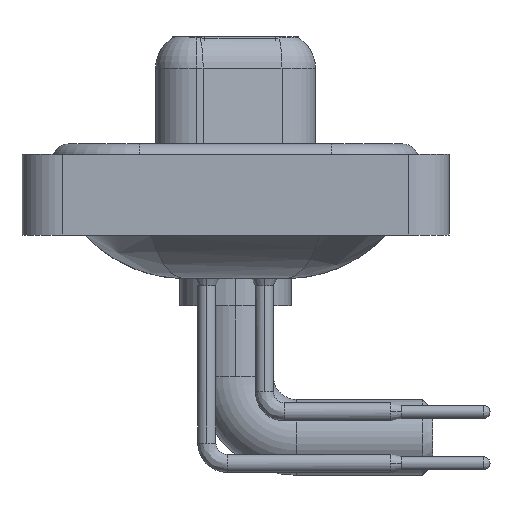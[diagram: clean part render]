
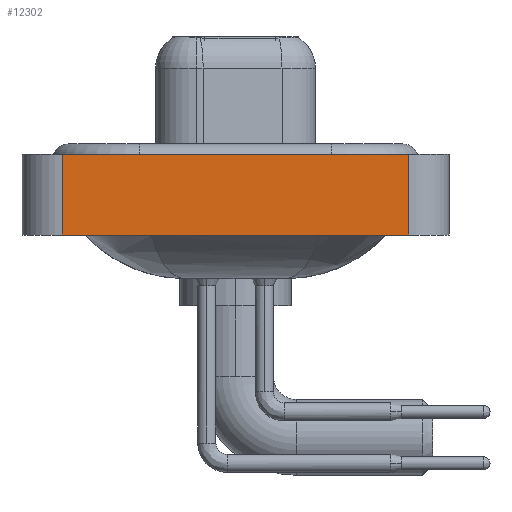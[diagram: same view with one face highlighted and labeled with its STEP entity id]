
A CAD part, left-side view. The second image highlights one B-rep face of the part: STEP entity #12302.
In plain terms, the highlighted planar face has unit normal (-1, 0, 0).
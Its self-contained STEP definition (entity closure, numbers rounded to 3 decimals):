
#582 = CARTESIAN_POINT ( 'NONE',  ( -7.3, 8.55, 0.4 ) ) ;
#676 = DIRECTION ( 'NONE',  ( -1., 0., 0. ) ) ;
#2109 = VERTEX_POINT ( 'NONE', #6338 ) ;
#2579 = LINE ( 'NONE', #5613, #11020 ) ;
#2845 = CARTESIAN_POINT ( 'NONE',  ( -7.3, 8.55, -3.6 ) ) ;
#2897 = CARTESIAN_POINT ( 'NONE',  ( -7.3, 8.55, -3.6 ) ) ;
#2934 = EDGE_CURVE ( 'NONE', #4146, #2109, #2579, .T. ) ;
#4146 = VERTEX_POINT ( 'NONE', #8092 ) ;
#4846 = EDGE_LOOP ( 'NONE', ( #12628, #10333, #7640, #14711 ) ) ;
#5613 = CARTESIAN_POINT ( 'NONE',  ( -7.3, -8.55, -3.6 ) ) ;
#5783 = VERTEX_POINT ( 'NONE', #582 ) ;
#6338 = CARTESIAN_POINT ( 'NONE',  ( -7.3, -8.55, 0.4 ) ) ;
#6369 = VECTOR ( 'NONE', #18248, 1000. ) ;
#7221 = DIRECTION ( 'NONE',  ( 0., -1., 0. ) ) ;
#7640 = ORIENTED_EDGE ( 'NONE', *, *, #9861, .F. ) ;
#8092 = CARTESIAN_POINT ( 'NONE',  ( -7.3, -8.55, -3.6 ) ) ;
#9240 = PLANE ( 'NONE',  #22042 ) ;
#9298 = LINE ( 'NONE', #19200, #12912 ) ;
#9682 = VECTOR ( 'NONE', #7221, 1000. ) ;
#9861 = EDGE_CURVE ( 'NONE', #12915, #5783, #14653, .T. ) ;
#10333 = ORIENTED_EDGE ( 'NONE', *, *, #17578, .F. ) ;
#11020 = VECTOR ( 'NONE', #14279, 1000. ) ;
#12300 = CARTESIAN_POINT ( 'NONE',  ( -7.3, -8.55, -3.6 ) ) ;
#12302 = ADVANCED_FACE ( 'NONE', ( #12826 ), #9240, .T. ) ;
#12628 = ORIENTED_EDGE ( 'NONE', *, *, #2934, .T. ) ;
#12826 = FACE_OUTER_BOUND ( 'NONE', #4846, .T. ) ;
#12912 = VECTOR ( 'NONE', #20601, 1000. ) ;
#12915 = VERTEX_POINT ( 'NONE', #2897 ) ;
#14279 = DIRECTION ( 'NONE',  ( 0., 0., 1. ) ) ;
#14653 = LINE ( 'NONE', #2845, #6369 ) ;
#14711 = ORIENTED_EDGE ( 'NONE', *, *, #19274, .T. ) ;
#15865 = DIRECTION ( 'NONE',  ( 0., 0., 1. ) ) ;
#16086 = CARTESIAN_POINT ( 'NONE',  ( -7.3, -8.55, -3.6 ) ) ;
#17578 = EDGE_CURVE ( 'NONE', #5783, #2109, #9298, .T. ) ;
#18248 = DIRECTION ( 'NONE',  ( 0., 0., 1. ) ) ;
#19200 = CARTESIAN_POINT ( 'NONE',  ( -7.3, -8.55, 0.4 ) ) ;
#19274 = EDGE_CURVE ( 'NONE', #12915, #4146, #20857, .T. ) ;
#20601 = DIRECTION ( 'NONE',  ( 0., -1., 0. ) ) ;
#20857 = LINE ( 'NONE', #12300, #9682 ) ;
#22042 = AXIS2_PLACEMENT_3D ( 'NONE', #16086, #676, #15865 ) ;
